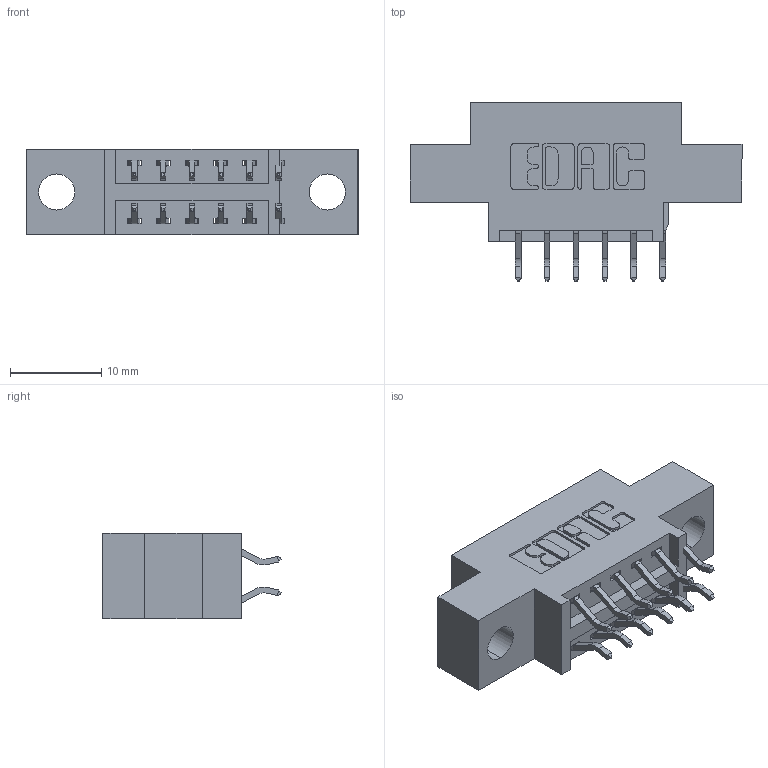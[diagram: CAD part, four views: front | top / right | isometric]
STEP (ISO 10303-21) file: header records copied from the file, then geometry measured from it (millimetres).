
FILE_DESCRIPTION (( 'STEP AP203' ), '1' );
FILE_NAME ('346-012-556-804.STEP', '2022-05-17T20:37:41', ( '' ), ( '' ), 'SwSTEP 2.0', 'SolidWorks 2020', '' );
FILE_SCHEMA (( 'CONFIG_CONTROL_DESIGN' ));
Length unit declared in the file: inch
Products named in the file (3): 346 Part_0.170 Offset - 0.156 Dia-TH; 345-292-001_556 Tail; 346-012-556-804
Assembly tree (13 placements, depth 2):
  346-012-556-804
    346 Part_0.170 Offset - 0.156 Dia-TH
    345-292-001_556 Tail  x12
Bounding box: 36.45 x 19.57 x 9.4 mm (x, y, z)
Volume: 3023.8 mm3; surface area: 3695 mm2
Topology: 13 solids, 13 shells, 824 faces, 2411 edges, 1590 vertices
Faces by surface type: plane 552, cylinder 272
Entity records: 9079 total; most frequent: CARTESIAN_POINT 1560, ORIENTED_EDGE 1478, DIRECTION 1415, EDGE_CURVE 739, VECTOR 579, LINE 579, VERTEX_POINT 490, AXIS2_PLACEMENT_3D 418
